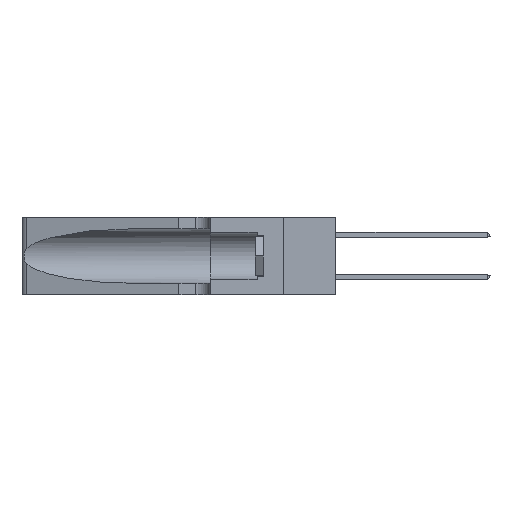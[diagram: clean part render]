
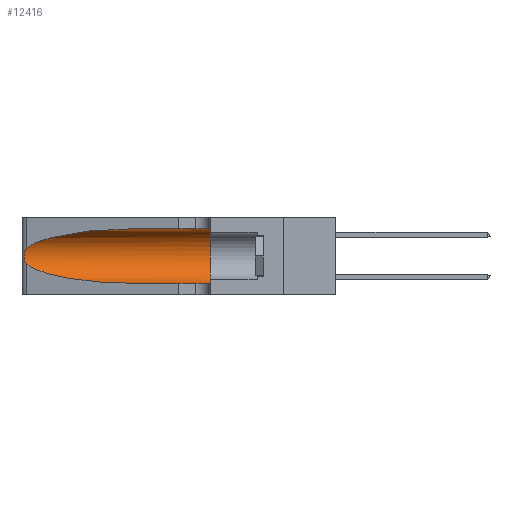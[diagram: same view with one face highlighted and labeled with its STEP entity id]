
A CAD part, left-side view. The second image highlights one B-rep face of the part: STEP entity #12416.
In plain terms, the highlighted cylindrical face has radius 3.308 mm (diameter 6.617 mm), a partial arc.
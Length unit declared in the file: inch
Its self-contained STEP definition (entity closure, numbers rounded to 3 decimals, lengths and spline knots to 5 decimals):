
#197 = DIRECTION ( 'NONE',  ( 0., -1., 0. ) ) ;
#826 = CARTESIAN_POINT ( 'NONE',  ( 0.1305, 0.72297, 0.31525 ) ) ;
#1014 = LINE ( 'NONE', #9228, #16170 ) ;
#2541 = VERTEX_POINT ( 'NONE', #7258 ) ;
#2822 = CARTESIAN_POINT ( 'NONE',  ( 0.25487, 1.22718, 0.14631 ) ) ;
#2890 = CARTESIAN_POINT ( 'NONE',  ( 0.25787, 1.23484, 0.2124 ) ) ;
#2993 = CARTESIAN_POINT ( 'NONE',  ( 0.25487, 1.22718, 0.14631 ) ) ;
#4745 = CIRCLE ( 'NONE', #7113, 0.13025 ) ;
#4768 = CARTESIAN_POINT ( 'NONE',  ( 0.1305, 0.72297, 0.05475 ) ) ;
#5800 = CARTESIAN_POINT ( 'NONE',  ( 0.25555, 1.22994, 0.2215 ) ) ;
#5932 = CARTESIAN_POINT ( 'NONE',  ( 0.26018, 1.23835, 0.19895 ) ) ;
#6145 = EDGE_CURVE ( 'NONE', #6728, #32847, #13626, .T. ) ;
#6215 = EDGE_CURVE ( 'NONE', #12086, #6376, #19516, .T. ) ;
#6376 = VERTEX_POINT ( 'NONE', #37067 ) ;
#6728 = VERTEX_POINT ( 'NONE', #2822 ) ;
#6922 = CARTESIAN_POINT ( 'NONE',  ( 0.25487, 1.22718, 0.22369 ) ) ;
#7113 = AXIS2_PLACEMENT_3D ( 'NONE', #26036, #8039, #29033 ) ;
#7258 = CARTESIAN_POINT ( 'NONE',  ( 0.25487, 1.22718, 0.22369 ) ) ;
#7899 = EDGE_CURVE ( 'NONE', #6376, #17595, #4745, .T. ) ;
#8039 = DIRECTION ( 'NONE',  ( 0., 1., 0. ) ) ;
#8981 = CARTESIAN_POINT ( 'NONE',  ( 0.26075, 1.23896, 0.178 ) ) ;
#9228 = CARTESIAN_POINT ( 'NONE',  ( 0.1305, 1.61858, 0.05475 ) ) ;
#10099 = DIRECTION ( 'NONE',  ( 0., 0., -1. ) ) ;
#11476 =( BOUNDED_CURVE ( )  B_SPLINE_CURVE ( 3, ( #826, #18923, #24949, #6922 ),
 .UNSPECIFIED., .F., .F. ) 
 B_SPLINE_CURVE_WITH_KNOTS ( ( 4, 4 ),
 ( 1.5708, 2.84003 ),
 .UNSPECIFIED. ) 
 CURVE ( )  GEOMETRIC_REPRESENTATION_ITEM ( )  RATIONAL_B_SPLINE_CURVE ( ( 1., 0.87, 0.87, 1. ) ) 
 REPRESENTATION_ITEM ( '' )  );
#11997 = CARTESIAN_POINT ( 'NONE',  ( 0.25856, 1.23593, 0.16098 ) ) ;
#12086 = VERTEX_POINT ( 'NONE', #17773 ) ;
#12416 = ADVANCED_FACE ( 'NONE', ( #19071 ), #26104, .F. ) ;
#13626 =( BOUNDED_CURVE ( )  B_SPLINE_CURVE ( 3, ( #2993, #21053, #18054, #24082 ),
 .UNSPECIFIED., .F., .F. ) 
 B_SPLINE_CURVE_WITH_KNOTS ( ( 4, 4 ),
 ( 3.44316, 4.71239 ),
 .UNSPECIFIED. ) 
 CURVE ( )  GEOMETRIC_REPRESENTATION_ITEM ( )  RATIONAL_B_SPLINE_CURVE ( ( 1., 0.87, 0.87, 1. ) ) 
 REPRESENTATION_ITEM ( '' )  );
#15062 = CARTESIAN_POINT ( 'NONE',  ( 0.25639, 1.23186, 0.15144 ) ) ;
#15289 = CARTESIAN_POINT ( 'NONE',  ( 0.1305, 1.61858, 0.31525 ) ) ;
#16170 = VECTOR ( 'NONE', #27064, 39.37008 ) ;
#17484 = ORIENTED_EDGE ( 'NONE', *, *, #7899, .F. ) ;
#17595 = VERTEX_POINT ( 'NONE', #25734 ) ;
#17773 = CARTESIAN_POINT ( 'NONE',  ( 0.1305, 0.72297, 0.31525 ) ) ;
#18054 = CARTESIAN_POINT ( 'NONE',  ( 0.18966, 0.96281, 0.05475 ) ) ;
#18073 = CARTESIAN_POINT ( 'NONE',  ( 0.25487, 1.22718, 0.14631 ) ) ;
#18923 = CARTESIAN_POINT ( 'NONE',  ( 0.18966, 0.96281, 0.31525 ) ) ;
#19071 = FACE_OUTER_BOUND ( 'NONE', #26979, .T. ) ;
#19516 = LINE ( 'NONE', #15289, #21380 ) ;
#19759 = ORIENTED_EDGE ( 'NONE', *, *, #26860, .T. ) ;
#20949 = CARTESIAN_POINT ( 'NONE',  ( 0.25639, 1.23184, 0.21858 ) ) ;
#21053 = CARTESIAN_POINT ( 'NONE',  ( 0.2373, 1.15595, 0.08982 ) ) ;
#21380 = VECTOR ( 'NONE', #197, 39.37008 ) ;
#22342 = AXIS2_PLACEMENT_3D ( 'NONE', #25209, #37043, #10099 ) ;
#23073 = ORIENTED_EDGE ( 'NONE', *, *, #37002, .T. ) ;
#23160 = B_SPLINE_CURVE_WITH_KNOTS ( 'NONE', 3,
 ( #35790, #5800, #20949, #2890, #23982, #5932, #26950, #8981, #29961, #11997, #32954, #15062, #35906, #18073 ),
 .UNSPECIFIED., .F., .F.,
 ( 4, 2, 2, 2, 2, 2, 4 ),
 ( 0., 0.00027, 0.00053, 0.00107, 0.0016, 0.00187, 0.00214 ),
 .UNSPECIFIED. ) ;
#23982 = CARTESIAN_POINT ( 'NONE',  ( 0.25854, 1.2359, 0.20912 ) ) ;
#24082 = CARTESIAN_POINT ( 'NONE',  ( 0.1305, 0.72297, 0.05475 ) ) ;
#24084 = EDGE_CURVE ( 'NONE', #12086, #2541, #11476, .T. ) ;
#24949 = CARTESIAN_POINT ( 'NONE',  ( 0.2373, 1.15595, 0.28018 ) ) ;
#25209 = CARTESIAN_POINT ( 'NONE',  ( 0.1305, 1.61858, 0.185 ) ) ;
#25734 = CARTESIAN_POINT ( 'NONE',  ( 0.1305, 0.35, 0.05475 ) ) ;
#26036 = CARTESIAN_POINT ( 'NONE',  ( 0.1305, 0.35, 0.185 ) ) ;
#26104 = CYLINDRICAL_SURFACE ( 'NONE', #22342, 0.13025 ) ;
#26860 = EDGE_CURVE ( 'NONE', #32847, #17595, #1014, .T. ) ;
#26950 = CARTESIAN_POINT ( 'NONE',  ( 0.26075, 1.23896, 0.19203 ) ) ;
#26979 = EDGE_LOOP ( 'NONE', ( #34830, #23073, #27888, #19759, #17484, #38093 ) ) ;
#27064 = DIRECTION ( 'NONE',  ( 0., -1., 0. ) ) ;
#27888 = ORIENTED_EDGE ( 'NONE', *, *, #6145, .T. ) ;
#29033 = DIRECTION ( 'NONE',  ( 0., 0., 1. ) ) ;
#29961 = CARTESIAN_POINT ( 'NONE',  ( 0.26017, 1.23833, 0.17102 ) ) ;
#32847 = VERTEX_POINT ( 'NONE', #4768 ) ;
#32954 = CARTESIAN_POINT ( 'NONE',  ( 0.25789, 1.23486, 0.15765 ) ) ;
#34830 = ORIENTED_EDGE ( 'NONE', *, *, #24084, .T. ) ;
#35790 = CARTESIAN_POINT ( 'NONE',  ( 0.25487, 1.22718, 0.22369 ) ) ;
#35906 = CARTESIAN_POINT ( 'NONE',  ( 0.25555, 1.22993, 0.14849 ) ) ;
#37002 = EDGE_CURVE ( 'NONE', #2541, #6728, #23160, .T. ) ;
#37043 = DIRECTION ( 'NONE',  ( 0., -1., 0. ) ) ;
#37067 = CARTESIAN_POINT ( 'NONE',  ( 0.1305, 0.35, 0.31525 ) ) ;
#38093 = ORIENTED_EDGE ( 'NONE', *, *, #6215, .F. ) ;
